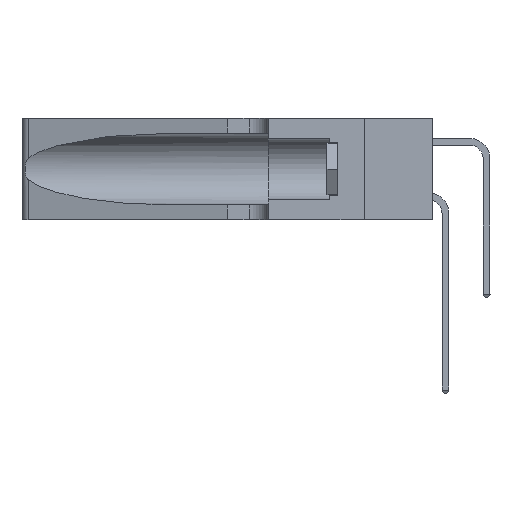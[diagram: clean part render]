
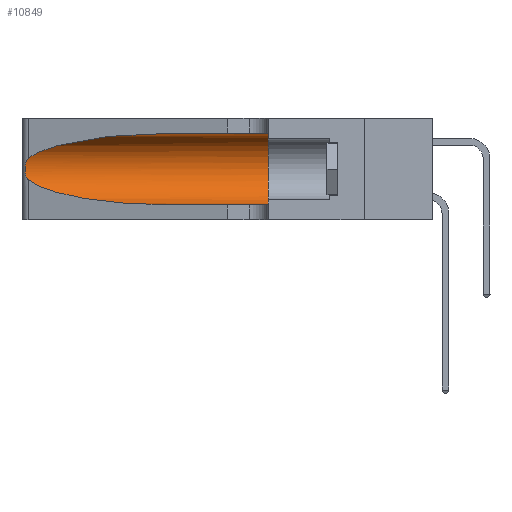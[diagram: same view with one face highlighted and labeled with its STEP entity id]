
A CAD part, left-side view. The second image highlights one B-rep face of the part: STEP entity #10849.
In plain terms, the highlighted cylindrical face has radius 3.308 mm (diameter 6.617 mm), a partial arc.
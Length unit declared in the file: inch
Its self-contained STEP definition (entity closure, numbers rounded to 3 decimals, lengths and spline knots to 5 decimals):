
#115 = CARTESIAN_POINT ( 'NONE',  ( 0.25487, 1.22718, 0.22369 ) ) ;
#186 = VERTEX_POINT ( 'NONE', #29340 ) ;
#1238 = CARTESIAN_POINT ( 'NONE',  ( 0.26017, 1.23833, 0.17102 ) ) ;
#1299 = CARTESIAN_POINT ( 'NONE',  ( 0.18966, 0.96281, 0.05475 ) ) ;
#1905 = ORIENTED_EDGE ( 'NONE', *, *, #16808, .T. ) ;
#2368 = VECTOR ( 'NONE', #4583, 39.37008 ) ;
#2796 = VERTEX_POINT ( 'NONE', #12516 ) ;
#2870 = EDGE_CURVE ( 'NONE', #27600, #6167, #25412, .T. ) ;
#3569 = CARTESIAN_POINT ( 'NONE',  ( 0.25789, 1.23486, 0.15765 ) ) ;
#3958 = DIRECTION ( 'NONE',  ( 0., -1., 0. ) ) ;
#4583 = DIRECTION ( 'NONE',  ( 0., -1., 0. ) ) ;
#4617 = DIRECTION ( 'NONE',  ( 0., -1., 0. ) ) ;
#5551 = ORIENTED_EDGE ( 'NONE', *, *, #17853, .T. ) ;
#5857 = CARTESIAN_POINT ( 'NONE',  ( 0.25487, 1.22718, 0.22369 ) ) ;
#5954 = CARTESIAN_POINT ( 'NONE',  ( 0.25555, 1.22993, 0.14849 ) ) ;
#6107 = LINE ( 'NONE', #29642, #22927 ) ;
#6167 = VERTEX_POINT ( 'NONE', #24520 ) ;
#6357 = CARTESIAN_POINT ( 'NONE',  ( 0.1305, 1.61858, 0.185 ) ) ;
#6895 = VERTEX_POINT ( 'NONE', #13258 ) ;
#6999 = VERTEX_POINT ( 'NONE', #20402 ) ;
#8211 = CARTESIAN_POINT ( 'NONE',  ( 0.25555, 1.22994, 0.2215 ) ) ;
#8651 = EDGE_CURVE ( 'NONE', #186, #6895, #26435, .T. ) ;
#9387 = CARTESIAN_POINT ( 'NONE',  ( 0.1305, 0.35, 0.185 ) ) ;
#10573 = CARTESIAN_POINT ( 'NONE',  ( 0.25787, 1.23484, 0.2124 ) ) ;
#10849 = ADVANCED_FACE ( 'NONE', ( #14009 ), #25273, .F. ) ;
#11735 = DIRECTION ( 'NONE',  ( 0., 0., 1. ) ) ;
#11790 = CARTESIAN_POINT ( 'NONE',  ( 0.1305, 0.72297, 0.31525 ) ) ;
#12351 = CARTESIAN_POINT ( 'NONE',  ( 0.25487, 1.22718, 0.22369 ) ) ;
#12516 = CARTESIAN_POINT ( 'NONE',  ( 0.1305, 0.72297, 0.05475 ) ) ;
#12898 = CARTESIAN_POINT ( 'NONE',  ( 0.26018, 1.23835, 0.19895 ) ) ;
#13258 = CARTESIAN_POINT ( 'NONE',  ( 0.1305, 0.35, 0.05475 ) ) ;
#13510 =( BOUNDED_CURVE ( )  B_SPLINE_CURVE ( 3, ( #11790, #25304, #14085, #115 ),
 .UNSPECIFIED., .F., .F. ) 
 B_SPLINE_CURVE_WITH_KNOTS ( ( 4, 4 ),
 ( 1.5708, 2.84003 ),
 .UNSPECIFIED. ) 
 CURVE ( )  GEOMETRIC_REPRESENTATION_ITEM ( )  RATIONAL_B_SPLINE_CURVE ( ( 1., 0.87, 0.87, 1. ) ) 
 REPRESENTATION_ITEM ( '' )  );
#14009 = FACE_OUTER_BOUND ( 'NONE', #27580, .T. ) ;
#14085 = CARTESIAN_POINT ( 'NONE',  ( 0.2373, 1.15595, 0.28018 ) ) ;
#14678 = ORIENTED_EDGE ( 'NONE', *, *, #28579, .T. ) ;
#15128 = CARTESIAN_POINT ( 'NONE',  ( 0.25487, 1.22718, 0.14631 ) ) ;
#15175 = CARTESIAN_POINT ( 'NONE',  ( 0.26075, 1.23896, 0.178 ) ) ;
#16642 =( BOUNDED_CURVE ( )  B_SPLINE_CURVE ( 3, ( #15128, #24181, #1299, #17497 ),
 .UNSPECIFIED., .F., .T. ) 
 B_SPLINE_CURVE_WITH_KNOTS ( ( 4, 4 ),
 ( 3.44316, 4.71239 ),
 .UNSPECIFIED. ) 
 CURVE ( )  GEOMETRIC_REPRESENTATION_ITEM ( )  RATIONAL_B_SPLINE_CURVE ( ( 1., 0.87, 0.87, 1. ) ) 
 REPRESENTATION_ITEM ( '' )  );
#16808 = EDGE_CURVE ( 'NONE', #6167, #2796, #16642, .T. ) ;
#17451 = CARTESIAN_POINT ( 'NONE',  ( 0.25856, 1.23593, 0.16098 ) ) ;
#17497 = CARTESIAN_POINT ( 'NONE',  ( 0.1305, 0.72297, 0.05475 ) ) ;
#17853 = EDGE_CURVE ( 'NONE', #6999, #27600, #13510, .T. ) ;
#17946 = AXIS2_PLACEMENT_3D ( 'NONE', #6357, #3958, #20117 ) ;
#19651 = CARTESIAN_POINT ( 'NONE',  ( 0.25639, 1.23184, 0.21858 ) ) ;
#19746 = CARTESIAN_POINT ( 'NONE',  ( 0.25639, 1.23186, 0.15144 ) ) ;
#20117 = DIRECTION ( 'NONE',  ( 0., 0., -1. ) ) ;
#20402 = CARTESIAN_POINT ( 'NONE',  ( 0.1305, 0.72297, 0.31525 ) ) ;
#20715 = CARTESIAN_POINT ( 'NONE',  ( 0.1305, 1.61858, 0.31525 ) ) ;
#20798 = LINE ( 'NONE', #20715, #2368 ) ;
#21998 = CARTESIAN_POINT ( 'NONE',  ( 0.25487, 1.22718, 0.14631 ) ) ;
#22927 = VECTOR ( 'NONE', #4617, 39.37008 ) ;
#23369 = AXIS2_PLACEMENT_3D ( 'NONE', #9387, #25248, #11735 ) ;
#24181 = CARTESIAN_POINT ( 'NONE',  ( 0.2373, 1.15595, 0.08982 ) ) ;
#24520 = CARTESIAN_POINT ( 'NONE',  ( 0.25487, 1.22718, 0.14631 ) ) ;
#25248 = DIRECTION ( 'NONE',  ( 0., 1., 0. ) ) ;
#25273 = CYLINDRICAL_SURFACE ( 'NONE', #17946, 0.13025 ) ;
#25304 = CARTESIAN_POINT ( 'NONE',  ( 0.18966, 0.96281, 0.31525 ) ) ;
#25412 = B_SPLINE_CURVE_WITH_KNOTS ( 'NONE', 3,
 ( #5857, #8211, #19651, #10573, #26393, #12898, #28642, #15175, #1238, #17451, #3569, #19746, #5954, #21998 ),
 .UNSPECIFIED., .F., .F.,
 ( 4, 2, 2, 2, 2, 2, 4 ),
 ( 0., 0.00027, 0.00053, 0.00107, 0.0016, 0.00187, 0.00214 ),
 .UNSPECIFIED. ) ;
#26393 = CARTESIAN_POINT ( 'NONE',  ( 0.25854, 1.2359, 0.20912 ) ) ;
#26435 = CIRCLE ( 'NONE', #23369, 0.13025 ) ;
#26731 = EDGE_CURVE ( 'NONE', #6999, #186, #20798, .T. ) ;
#27440 = ORIENTED_EDGE ( 'NONE', *, *, #8651, .F. ) ;
#27580 = EDGE_LOOP ( 'NONE', ( #5551, #28450, #1905, #14678, #27440, #28170 ) ) ;
#27600 = VERTEX_POINT ( 'NONE', #12351 ) ;
#28170 = ORIENTED_EDGE ( 'NONE', *, *, #26731, .F. ) ;
#28450 = ORIENTED_EDGE ( 'NONE', *, *, #2870, .T. ) ;
#28579 = EDGE_CURVE ( 'NONE', #2796, #6895, #6107, .T. ) ;
#28642 = CARTESIAN_POINT ( 'NONE',  ( 0.26075, 1.23896, 0.19203 ) ) ;
#29340 = CARTESIAN_POINT ( 'NONE',  ( 0.1305, 0.35, 0.31525 ) ) ;
#29642 = CARTESIAN_POINT ( 'NONE',  ( 0.1305, 1.61858, 0.05475 ) ) ;
